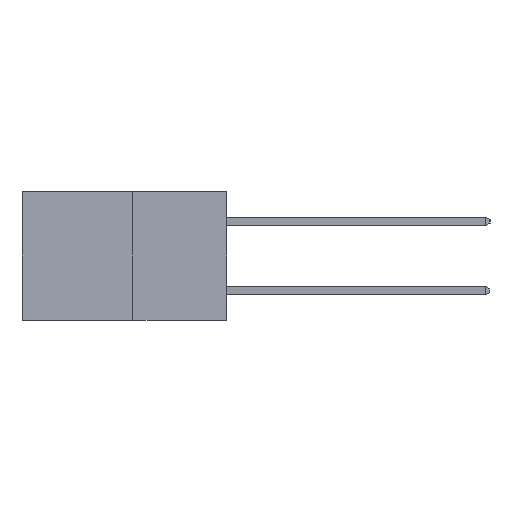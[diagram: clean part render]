
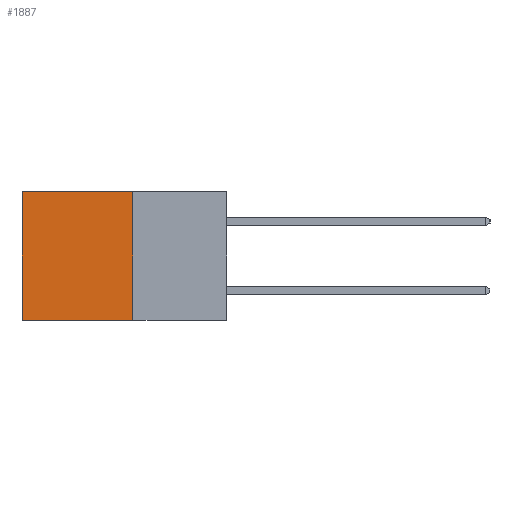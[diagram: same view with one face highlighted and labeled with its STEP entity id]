
A CAD part, left-side view. The second image highlights one B-rep face of the part: STEP entity #1887.
In plain terms, the highlighted planar face has unit normal (-1, 0, 0).
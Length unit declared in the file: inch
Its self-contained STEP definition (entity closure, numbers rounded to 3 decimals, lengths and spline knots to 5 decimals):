
#12 = LINE ( 'NONE', #5797, #1844 ) ;
#91 = CARTESIAN_POINT ( 'NONE',  ( 0.277, 0.59, -0.37 ) ) ;
#1315 = VECTOR ( 'NONE', #7773, 39.37008 ) ;
#1491 = LINE ( 'NONE', #8779, #9694 ) ;
#1758 = CARTESIAN_POINT ( 'NONE',  ( 0.277, 0.59, -0.37 ) ) ;
#1844 = VECTOR ( 'NONE', #6640, 39.37008 ) ;
#1887 = ADVANCED_FACE ( 'NONE', ( #4377 ), #10368, .F. ) ;
#2055 = AXIS2_PLACEMENT_3D ( 'NONE', #10452, #10326, #10313 ) ;
#2174 = LINE ( 'NONE', #9669, #10488 ) ;
#2194 = DIRECTION ( 'NONE',  ( 0., 1., 0. ) ) ;
#2945 = CARTESIAN_POINT ( 'NONE',  ( 0.277, 0.27, -0.37 ) ) ;
#3652 = LINE ( 'NONE', #91, #1315 ) ;
#3971 = ORIENTED_EDGE ( 'NONE', *, *, #8728, .T. ) ;
#4088 = ORIENTED_EDGE ( 'NONE', *, *, #10117, .F. ) ;
#4156 = CARTESIAN_POINT ( 'NONE',  ( 0.277, 0.27, 0. ) ) ;
#4242 = VERTEX_POINT ( 'NONE', #1758 ) ;
#4377 = FACE_OUTER_BOUND ( 'NONE', #4560, .T. ) ;
#4560 = EDGE_LOOP ( 'NONE', ( #3971, #4088, #7220, #7338 ) ) ;
#4808 = VERTEX_POINT ( 'NONE', #4156 ) ;
#5203 = VERTEX_POINT ( 'NONE', #2945 ) ;
#5462 = VERTEX_POINT ( 'NONE', #6669 ) ;
#5797 = CARTESIAN_POINT ( 'NONE',  ( 0.277, 0.27, -0.37 ) ) ;
#6640 = DIRECTION ( 'NONE',  ( 0., 1., 0. ) ) ;
#6669 = CARTESIAN_POINT ( 'NONE',  ( 0.277, 0.59, 0. ) ) ;
#7220 = ORIENTED_EDGE ( 'NONE', *, *, #7627, .F. ) ;
#7338 = ORIENTED_EDGE ( 'NONE', *, *, #7445, .T. ) ;
#7445 = EDGE_CURVE ( 'NONE', #4808, #5462, #1491, .T. ) ;
#7627 = EDGE_CURVE ( 'NONE', #4808, #5203, #2174, .T. ) ;
#7773 = DIRECTION ( 'NONE',  ( 0., 0., -1. ) ) ;
#8728 = EDGE_CURVE ( 'NONE', #5462, #4242, #3652, .T. ) ;
#8779 = CARTESIAN_POINT ( 'NONE',  ( 0.277, 0.27, 0. ) ) ;
#9669 = CARTESIAN_POINT ( 'NONE',  ( 0.277, 0.27, -0.37 ) ) ;
#9694 = VECTOR ( 'NONE', #2194, 39.37008 ) ;
#10117 = EDGE_CURVE ( 'NONE', #5203, #4242, #12, .T. ) ;
#10313 = DIRECTION ( 'NONE',  ( 0., 0., -1. ) ) ;
#10326 = DIRECTION ( 'NONE',  ( 1., 0., 0. ) ) ;
#10368 = PLANE ( 'NONE',  #2055 ) ;
#10437 = DIRECTION ( 'NONE',  ( 0., 0., -1. ) ) ;
#10452 = CARTESIAN_POINT ( 'NONE',  ( 0.277, 0.27, -0.37 ) ) ;
#10488 = VECTOR ( 'NONE', #10437, 39.37008 ) ;
